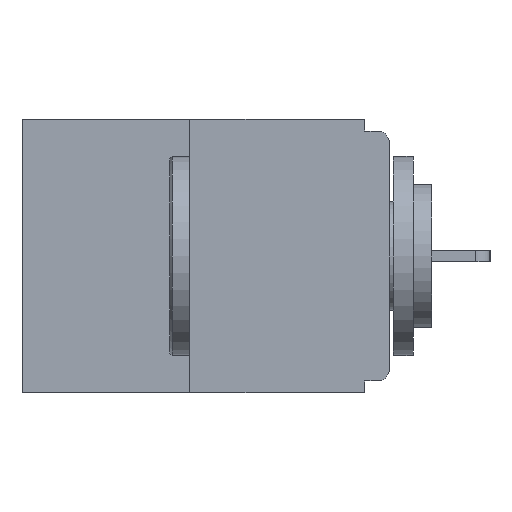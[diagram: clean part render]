
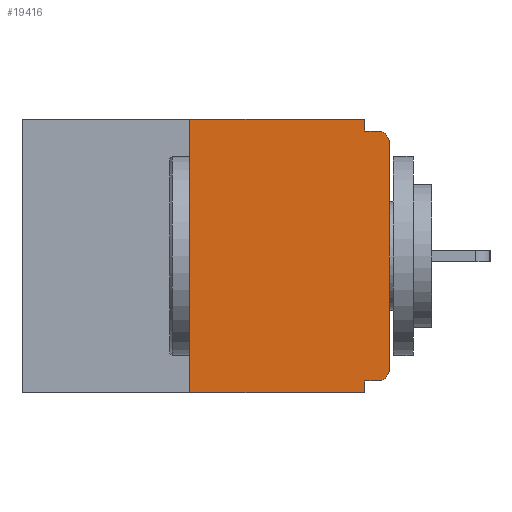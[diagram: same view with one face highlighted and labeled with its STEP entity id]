
A CAD part, left-side view. The second image highlights one B-rep face of the part: STEP entity #19416.
In plain terms, the highlighted planar face has unit normal (-1, 0, 0).
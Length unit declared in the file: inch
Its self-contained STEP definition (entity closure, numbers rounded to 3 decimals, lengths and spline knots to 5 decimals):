
#122 = DIRECTION ( 'NONE',  ( 0., -1., 0. ) ) ;
#313 = CARTESIAN_POINT ( 'NONE',  ( 0., 0.031, -0.015 ) ) ;
#368 = EDGE_CURVE ( 'NONE', #3695, #15098, #22316, .T. ) ;
#652 = DIRECTION ( 'NONE',  ( 0., -1., 0. ) ) ;
#718 = DIRECTION ( 'NONE',  ( 0., -1., 0. ) ) ;
#1032 = LINE ( 'NONE', #4492, #17596 ) ;
#1346 = CARTESIAN_POINT ( 'NONE',  ( 0., 0.015, -0.313 ) ) ;
#1349 = EDGE_CURVE ( 'NONE', #22150, #19150, #16292, .T. ) ;
#2377 = LINE ( 'NONE', #14990, #17316 ) ;
#2424 = LINE ( 'NONE', #9620, #13144 ) ;
#2789 = DIRECTION ( 'NONE',  ( 0., 0., -1. ) ) ;
#3068 = CARTESIAN_POINT ( 'NONE',  ( 0., 0.015, -0.328 ) ) ;
#3695 = VERTEX_POINT ( 'NONE', #11548 ) ;
#3698 = EDGE_CURVE ( 'NONE', #11273, #3695, #1032, .T. ) ;
#3841 = ORIENTED_EDGE ( 'NONE', *, *, #1349, .F. ) ;
#3917 = CARTESIAN_POINT ( 'NONE',  ( 0., 0.031, -0.343 ) ) ;
#4030 = AXIS2_PLACEMENT_3D ( 'NONE', #1346, #15136, #22611 ) ;
#4145 = CARTESIAN_POINT ( 'NONE',  ( 0., 0., -0.03 ) ) ;
#4492 = CARTESIAN_POINT ( 'NONE',  ( 0., 0., -0.328 ) ) ;
#4523 = CARTESIAN_POINT ( 'NONE',  ( 0., 0.46, 0. ) ) ;
#4828 = CARTESIAN_POINT ( 'NONE',  ( 0., 0.25, 0. ) ) ;
#5111 = VERTEX_POINT ( 'NONE', #4828 ) ;
#5392 = AXIS2_PLACEMENT_3D ( 'NONE', #4523, #8613, #19321 ) ;
#5532 = CIRCLE ( 'NONE', #4030, 0.015 ) ;
#6149 = ORIENTED_EDGE ( 'NONE', *, *, #19818, .T. ) ;
#6386 = DIRECTION ( 'NONE',  ( -1., 0., 0. ) ) ;
#6532 = DIRECTION ( 'NONE',  ( 0., 0., 1. ) ) ;
#7941 = CARTESIAN_POINT ( 'NONE',  ( 0., 0.031, -0.343 ) ) ;
#8613 = DIRECTION ( 'NONE',  ( 1., 0., 0. ) ) ;
#9620 = CARTESIAN_POINT ( 'NONE',  ( 0., 0.46, -0.343 ) ) ;
#9972 = CARTESIAN_POINT ( 'NONE',  ( 0., 0.25, -0.343 ) ) ;
#10462 = ORIENTED_EDGE ( 'NONE', *, *, #3698, .F. ) ;
#10890 = CARTESIAN_POINT ( 'NONE',  ( 0., 0.015, -0.015 ) ) ;
#11003 = ORIENTED_EDGE ( 'NONE', *, *, #16442, .T. ) ;
#11273 = VERTEX_POINT ( 'NONE', #3068 ) ;
#11541 = EDGE_CURVE ( 'NONE', #13099, #15098, #2424, .T. ) ;
#11548 = CARTESIAN_POINT ( 'NONE',  ( 0., 0.031, -0.328 ) ) ;
#11620 = CIRCLE ( 'NONE', #14981, 0.015 ) ;
#11631 = CARTESIAN_POINT ( 'NONE',  ( 0., 0.25, 0. ) ) ;
#11685 = EDGE_CURVE ( 'NONE', #22527, #22150, #21175, .T. ) ;
#12166 = PLANE ( 'NONE',  #5392 ) ;
#12252 = ORIENTED_EDGE ( 'NONE', *, *, #11541, .T. ) ;
#12323 = ORIENTED_EDGE ( 'NONE', *, *, #13134, .T. ) ;
#12334 = ORIENTED_EDGE ( 'NONE', *, *, #16614, .F. ) ;
#12438 = EDGE_CURVE ( 'NONE', #5111, #22527, #2377, .T. ) ;
#12564 = VERTEX_POINT ( 'NONE', #4145 ) ;
#13099 = VERTEX_POINT ( 'NONE', #9972 ) ;
#13134 = EDGE_CURVE ( 'NONE', #11273, #23000, #5532, .T. ) ;
#13144 = VECTOR ( 'NONE', #652, 39.37008 ) ;
#13452 = ORIENTED_EDGE ( 'NONE', *, *, #12438, .F. ) ;
#14067 = VECTOR ( 'NONE', #122, 39.37008 ) ;
#14981 = AXIS2_PLACEMENT_3D ( 'NONE', #20772, #6386, #20886 ) ;
#14989 = ORIENTED_EDGE ( 'NONE', *, *, #368, .F. ) ;
#14990 = CARTESIAN_POINT ( 'NONE',  ( 0., 0.46, 0. ) ) ;
#15098 = VERTEX_POINT ( 'NONE', #7941 ) ;
#15136 = DIRECTION ( 'NONE',  ( -1., 0., 0. ) ) ;
#15303 = CARTESIAN_POINT ( 'NONE',  ( 0., 0., -0.313 ) ) ;
#15448 = CARTESIAN_POINT ( 'NONE',  ( 0., 0.031, 0. ) ) ;
#15733 = VECTOR ( 'NONE', #6532, 39.37008 ) ;
#16292 = LINE ( 'NONE', #19485, #14067 ) ;
#16442 = EDGE_CURVE ( 'NONE', #12564, #19150, #11620, .T. ) ;
#16614 = EDGE_CURVE ( 'NONE', #13099, #5111, #17144, .T. ) ;
#16728 = DIRECTION ( 'NONE',  ( 0., 0., -1. ) ) ;
#16954 = DIRECTION ( 'NONE',  ( 0., 1., 0. ) ) ;
#16955 = DIRECTION ( 'NONE',  ( 0., 0., 1. ) ) ;
#17144 = LINE ( 'NONE', #11631, #15733 ) ;
#17316 = VECTOR ( 'NONE', #718, 39.37008 ) ;
#17347 = FACE_OUTER_BOUND ( 'NONE', #20726, .T. ) ;
#17596 = VECTOR ( 'NONE', #16954, 39.37008 ) ;
#18334 = VECTOR ( 'NONE', #16728, 39.37008 ) ;
#18413 = VECTOR ( 'NONE', #2789, 39.37008 ) ;
#19150 = VERTEX_POINT ( 'NONE', #10890 ) ;
#19321 = DIRECTION ( 'NONE',  ( 0., 0., -1. ) ) ;
#19416 = ADVANCED_FACE ( 'NONE', ( #17347 ), #12166, .F. ) ;
#19485 = CARTESIAN_POINT ( 'NONE',  ( 0., 0., -0.015 ) ) ;
#19818 = EDGE_CURVE ( 'NONE', #23000, #12564, #22376, .T. ) ;
#20613 = CARTESIAN_POINT ( 'NONE',  ( 0., 0., 0. ) ) ;
#20726 = EDGE_LOOP ( 'NONE', ( #13452, #12334, #12252, #14989, #10462, #12323, #6149, #11003, #3841, #20956 ) ) ;
#20772 = CARTESIAN_POINT ( 'NONE',  ( 0., 0.015, -0.03 ) ) ;
#20886 = DIRECTION ( 'NONE',  ( 0., 0., -1. ) ) ;
#20956 = ORIENTED_EDGE ( 'NONE', *, *, #11685, .F. ) ;
#21175 = LINE ( 'NONE', #22617, #18413 ) ;
#21606 = VECTOR ( 'NONE', #16955, 39.37008 ) ;
#22150 = VERTEX_POINT ( 'NONE', #313 ) ;
#22316 = LINE ( 'NONE', #3917, #18334 ) ;
#22376 = LINE ( 'NONE', #20613, #21606 ) ;
#22527 = VERTEX_POINT ( 'NONE', #15448 ) ;
#22611 = DIRECTION ( 'NONE',  ( 0., 0., -1. ) ) ;
#22617 = CARTESIAN_POINT ( 'NONE',  ( 0., 0.031, 0. ) ) ;
#23000 = VERTEX_POINT ( 'NONE', #15303 ) ;
